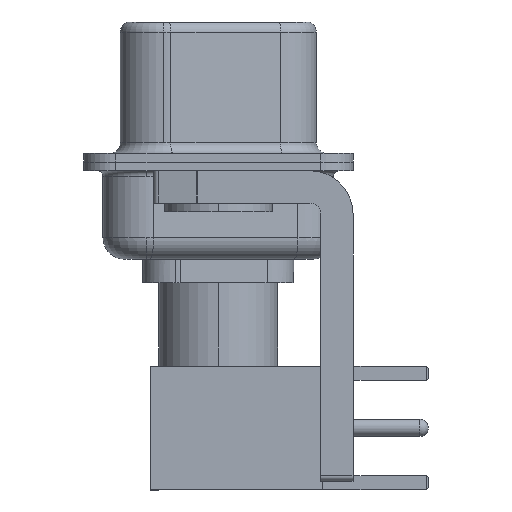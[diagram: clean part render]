
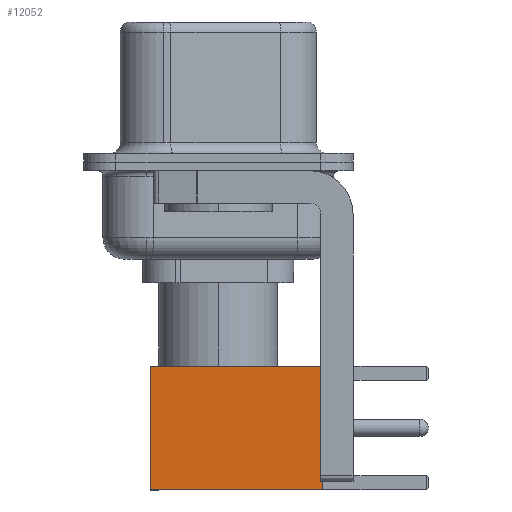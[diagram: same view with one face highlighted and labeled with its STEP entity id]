
A CAD part, left-side view. The second image highlights one B-rep face of the part: STEP entity #12052.
In plain terms, the highlighted face is planar.
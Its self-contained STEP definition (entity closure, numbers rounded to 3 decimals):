
#1237 = CARTESIAN_POINT ( 'NONE',  ( 2.875, 2.875, 0. ) ) ;
#1438 = VERTEX_POINT ( 'NONE', #13286 ) ;
#1661 = AXIS2_PLACEMENT_3D ( 'NONE', #1237, #2411, #7686 ) ;
#1734 = LINE ( 'NONE', #6838, #16052 ) ;
#1774 = CARTESIAN_POINT ( 'NONE',  ( 0., 2.875, 0. ) ) ;
#1934 = ORIENTED_EDGE ( 'NONE', *, *, #13361, .F. ) ;
#2207 = DIRECTION ( 'NONE',  ( 0., 0., -1. ) ) ;
#2262 = CARTESIAN_POINT ( 'NONE',  ( -2.875, 2.875, 0. ) ) ;
#2411 = DIRECTION ( 'NONE',  ( 0., 1., 0. ) ) ;
#3105 = CARTESIAN_POINT ( 'NONE',  ( -2.875, 2.875, 8. ) ) ;
#3192 = VECTOR ( 'NONE', #2207, 1000. ) ;
#4457 = DIRECTION ( 'NONE',  ( -1., 0., 0. ) ) ;
#4904 = LINE ( 'NONE', #15137, #3192 ) ;
#5179 = VECTOR ( 'NONE', #4457, 1000. ) ;
#5820 = DIRECTION ( 'NONE',  ( -1., 0., 0. ) ) ;
#6838 = CARTESIAN_POINT ( 'NONE',  ( 0., 2.875, 8. ) ) ;
#6989 = EDGE_CURVE ( 'NONE', #10974, #1438, #4904, .T. ) ;
#7022 = EDGE_CURVE ( 'NONE', #10974, #7712, #1734, .T. ) ;
#7112 = DIRECTION ( 'NONE',  ( 0., 0., -1. ) ) ;
#7686 = DIRECTION ( 'NONE',  ( 0., 0., 1. ) ) ;
#7712 = VERTEX_POINT ( 'NONE', #3105 ) ;
#9485 = LINE ( 'NONE', #1774, #5179 ) ;
#10289 = PLANE ( 'NONE',  #1661 ) ;
#10571 = EDGE_LOOP ( 'NONE', ( #12187, #11666, #1934, #11885 ) ) ;
#10968 = VERTEX_POINT ( 'NONE', #2262 ) ;
#10974 = VERTEX_POINT ( 'NONE', #11552 ) ;
#11552 = CARTESIAN_POINT ( 'NONE',  ( 2.875, 2.875, 8. ) ) ;
#11666 = ORIENTED_EDGE ( 'NONE', *, *, #15563, .T. ) ;
#11885 = ORIENTED_EDGE ( 'NONE', *, *, #7022, .F. ) ;
#12052 = ADVANCED_FACE ( 'NONE', ( #15174 ), #10289, .T. ) ;
#12187 = ORIENTED_EDGE ( 'NONE', *, *, #6989, .T. ) ;
#13286 = CARTESIAN_POINT ( 'NONE',  ( 2.875, 2.875, 0. ) ) ;
#13361 = EDGE_CURVE ( 'NONE', #7712, #10968, #14759, .T. ) ;
#13501 = CARTESIAN_POINT ( 'NONE',  ( -2.875, 2.875, 0. ) ) ;
#14759 = LINE ( 'NONE', #13501, #15640 ) ;
#15137 = CARTESIAN_POINT ( 'NONE',  ( 2.875, 2.875, 0. ) ) ;
#15174 = FACE_OUTER_BOUND ( 'NONE', #10571, .T. ) ;
#15563 = EDGE_CURVE ( 'NONE', #1438, #10968, #9485, .T. ) ;
#15640 = VECTOR ( 'NONE', #7112, 1000. ) ;
#16052 = VECTOR ( 'NONE', #5820, 1000. ) ;
